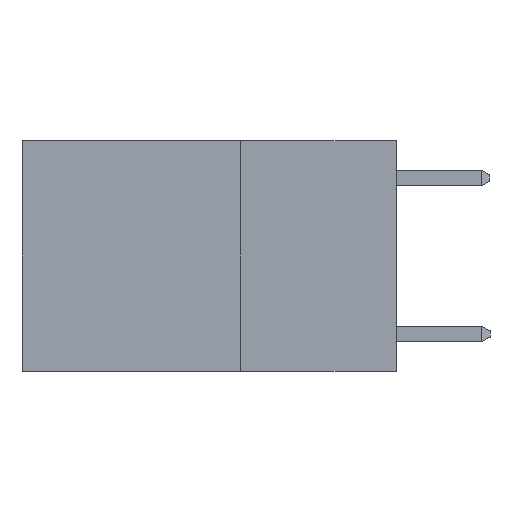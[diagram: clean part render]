
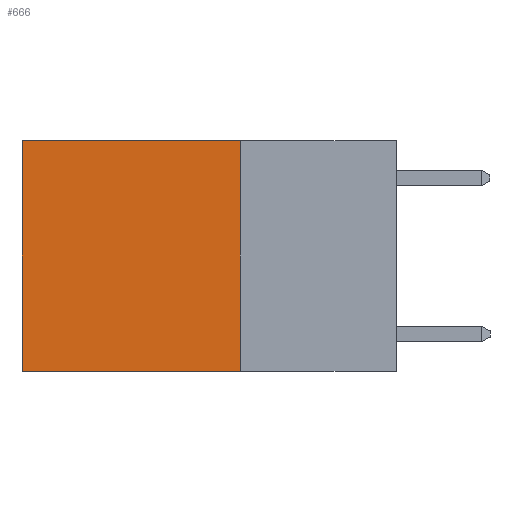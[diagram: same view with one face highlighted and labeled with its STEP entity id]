
A CAD part, left-side view. The second image highlights one B-rep face of the part: STEP entity #666.
In plain terms, the highlighted planar face has unit normal (-1, 0, 0).
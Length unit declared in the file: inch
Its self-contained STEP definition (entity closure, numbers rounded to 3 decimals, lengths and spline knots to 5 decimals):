
#65 = CARTESIAN_POINT ( 'NONE',  ( 0.2625, 0.6, 0. ) ) ;
#85 = CARTESIAN_POINT ( 'NONE',  ( 0.2625, 0.25, 0. ) ) ;
#217 = DIRECTION ( 'NONE',  ( 0., 0., -1. ) ) ;
#650 = VERTEX_POINT ( 'NONE', #823 ) ;
#666 = ADVANCED_FACE ( 'NONE', ( #8264 ), #4015, .F. ) ;
#823 = CARTESIAN_POINT ( 'NONE',  ( 0.2625, 0.25, -0.37 ) ) ;
#935 = CARTESIAN_POINT ( 'NONE',  ( 0.2625, 0.25, -0.37 ) ) ;
#1277 = VECTOR ( 'NONE', #1617, 39.37008 ) ;
#1609 = DIRECTION ( 'NONE',  ( 1., 0., 0. ) ) ;
#1617 = DIRECTION ( 'NONE',  ( 0., 1., 0. ) ) ;
#2736 = VERTEX_POINT ( 'NONE', #8024 ) ;
#2880 = DIRECTION ( 'NONE',  ( 0., 0., -1. ) ) ;
#2904 = VECTOR ( 'NONE', #217, 39.37008 ) ;
#3560 = DIRECTION ( 'NONE',  ( 0., 0., -1. ) ) ;
#3668 = EDGE_CURVE ( 'NONE', #650, #7463, #4718, .T. ) ;
#3944 = ORIENTED_EDGE ( 'NONE', *, *, #4481, .F. ) ;
#4015 = PLANE ( 'NONE',  #6406 ) ;
#4105 = CARTESIAN_POINT ( 'NONE',  ( 0.2625, 0.25, 0. ) ) ;
#4397 = EDGE_CURVE ( 'NONE', #2736, #6157, #5117, .T. ) ;
#4481 = EDGE_CURVE ( 'NONE', #2736, #650, #4719, .T. ) ;
#4566 = LINE ( 'NONE', #5418, #2904 ) ;
#4718 = LINE ( 'NONE', #935, #1277 ) ;
#4719 = LINE ( 'NONE', #6115, #7878 ) ;
#5117 = LINE ( 'NONE', #4105, #6696 ) ;
#5418 = CARTESIAN_POINT ( 'NONE',  ( 0.2625, 0.6, 0. ) ) ;
#6115 = CARTESIAN_POINT ( 'NONE',  ( 0.2625, 0.25, 0. ) ) ;
#6157 = VERTEX_POINT ( 'NONE', #65 ) ;
#6406 = AXIS2_PLACEMENT_3D ( 'NONE', #85, #1609, #2880 ) ;
#6696 = VECTOR ( 'NONE', #8128, 39.37008 ) ;
#6810 = ORIENTED_EDGE ( 'NONE', *, *, #3668, .F. ) ;
#6903 = CARTESIAN_POINT ( 'NONE',  ( 0.2625, 0.6, -0.37 ) ) ;
#7367 = EDGE_CURVE ( 'NONE', #6157, #7463, #4566, .T. ) ;
#7463 = VERTEX_POINT ( 'NONE', #6903 ) ;
#7724 = EDGE_LOOP ( 'NONE', ( #8463, #6810, #3944, #8101 ) ) ;
#7878 = VECTOR ( 'NONE', #3560, 39.37008 ) ;
#8024 = CARTESIAN_POINT ( 'NONE',  ( 0.2625, 0.25, 0. ) ) ;
#8101 = ORIENTED_EDGE ( 'NONE', *, *, #4397, .T. ) ;
#8128 = DIRECTION ( 'NONE',  ( 0., 1., 0. ) ) ;
#8264 = FACE_OUTER_BOUND ( 'NONE', #7724, .T. ) ;
#8463 = ORIENTED_EDGE ( 'NONE', *, *, #7367, .T. ) ;
